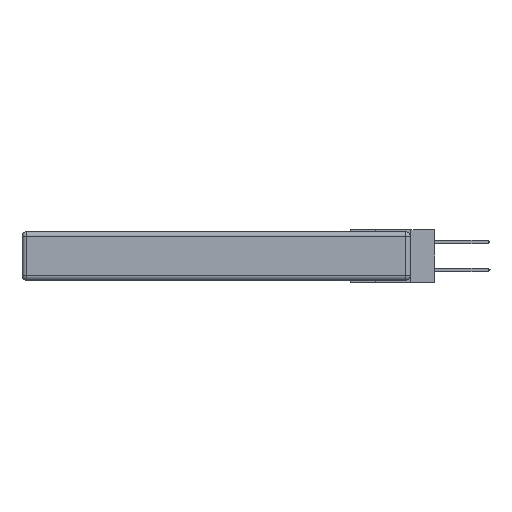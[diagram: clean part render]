
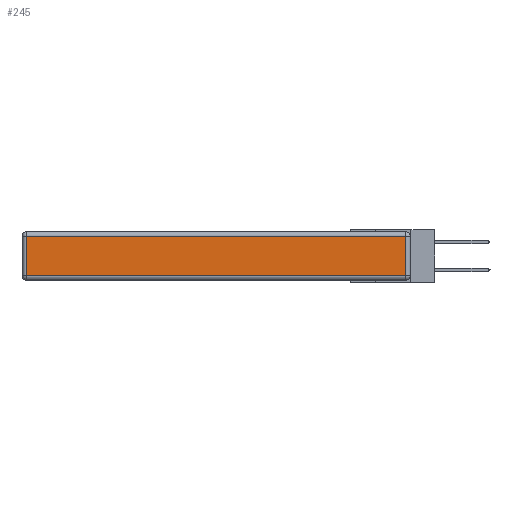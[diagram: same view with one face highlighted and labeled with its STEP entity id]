
A CAD part, left-side view. The second image highlights one B-rep face of the part: STEP entity #245.
In plain terms, the highlighted planar face has unit normal (-1, 0, 0).
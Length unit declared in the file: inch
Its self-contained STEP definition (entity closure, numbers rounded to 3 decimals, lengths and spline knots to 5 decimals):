
#245 = ADVANCED_FACE ( 'NONE', ( #15979 ), #10738, .T. ) ;
#595 = CARTESIAN_POINT ( 'NONE',  ( 0., 2.72, -0.03 ) ) ;
#823 = DIRECTION ( 'NONE',  ( 0., -1., 0. ) ) ;
#1129 = CARTESIAN_POINT ( 'NONE',  ( 0., 2.75, -0.03 ) ) ;
#1320 = VECTOR ( 'NONE', #6809, 39.37008 ) ;
#1477 = VERTEX_POINT ( 'NONE', #595 ) ;
#1528 = LINE ( 'NONE', #8189, #1320 ) ;
#1965 = VERTEX_POINT ( 'NONE', #5068 ) ;
#3565 = VERTEX_POINT ( 'NONE', #4801 ) ;
#3600 = VECTOR ( 'NONE', #9303, 39.37008 ) ;
#4514 = VECTOR ( 'NONE', #10351, 39.37008 ) ;
#4641 = AXIS2_PLACEMENT_3D ( 'NONE', #16151, #5481, #14668 ) ;
#4660 = VECTOR ( 'NONE', #823, 39.37008 ) ;
#4801 = CARTESIAN_POINT ( 'NONE',  ( 0., 2.72, -0.313 ) ) ;
#5068 = CARTESIAN_POINT ( 'NONE',  ( 0., 0.03, -0.03 ) ) ;
#5481 = DIRECTION ( 'NONE',  ( -1., 0., 0. ) ) ;
#6004 = LINE ( 'NONE', #1129, #4514 ) ;
#6809 = DIRECTION ( 'NONE',  ( 0., 0., 1. ) ) ;
#8189 = CARTESIAN_POINT ( 'NONE',  ( 0., 0.03, -0.343 ) ) ;
#8297 = LINE ( 'NONE', #13201, #4660 ) ;
#9303 = DIRECTION ( 'NONE',  ( 0., 0., -1. ) ) ;
#9743 = EDGE_CURVE ( 'NONE', #1477, #3565, #13330, .T. ) ;
#10196 = EDGE_CURVE ( 'NONE', #3565, #10933, #8297, .T. ) ;
#10351 = DIRECTION ( 'NONE',  ( 0., 1., 0. ) ) ;
#10738 = PLANE ( 'NONE',  #4641 ) ;
#10867 = ORIENTED_EDGE ( 'NONE', *, *, #10196, .T. ) ;
#10933 = VERTEX_POINT ( 'NONE', #14429 ) ;
#11198 = ORIENTED_EDGE ( 'NONE', *, *, #13173, .T. ) ;
#13173 = EDGE_CURVE ( 'NONE', #1965, #1477, #6004, .T. ) ;
#13201 = CARTESIAN_POINT ( 'NONE',  ( 0., 0., -0.313 ) ) ;
#13273 = EDGE_LOOP ( 'NONE', ( #10867, #15146, #11198, #14097 ) ) ;
#13330 = LINE ( 'NONE', #17296, #3600 ) ;
#13840 = EDGE_CURVE ( 'NONE', #10933, #1965, #1528, .T. ) ;
#14097 = ORIENTED_EDGE ( 'NONE', *, *, #9743, .T. ) ;
#14429 = CARTESIAN_POINT ( 'NONE',  ( 0., 0.03, -0.313 ) ) ;
#14668 = DIRECTION ( 'NONE',  ( 0., 0., 1. ) ) ;
#15146 = ORIENTED_EDGE ( 'NONE', *, *, #13840, .T. ) ;
#15979 = FACE_OUTER_BOUND ( 'NONE', #13273, .T. ) ;
#16151 = CARTESIAN_POINT ( 'NONE',  ( 0., 0., -0.343 ) ) ;
#17296 = CARTESIAN_POINT ( 'NONE',  ( 0., 2.72, -0.343 ) ) ;
